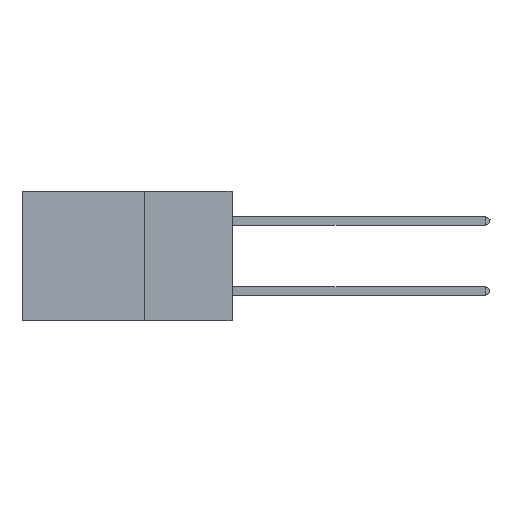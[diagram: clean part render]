
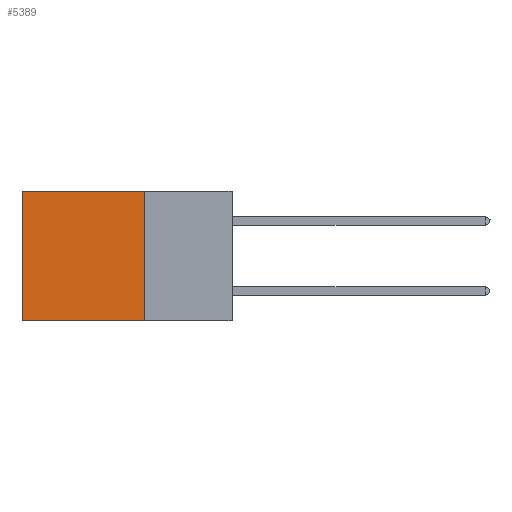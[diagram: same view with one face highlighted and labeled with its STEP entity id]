
A CAD part, left-side view. The second image highlights one B-rep face of the part: STEP entity #5389.
In plain terms, the highlighted planar face has unit normal (-1, 0, 0).
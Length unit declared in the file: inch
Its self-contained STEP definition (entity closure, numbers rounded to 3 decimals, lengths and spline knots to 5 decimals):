
#2320 = LINE ( 'NONE', #43540, #10489 ) ;
#3281 = DIRECTION ( 'NONE',  ( 0., 1., 0. ) ) ;
#3427 = FACE_OUTER_BOUND ( 'NONE', #35439, .T. ) ;
#4318 = VERTEX_POINT ( 'NONE', #36390 ) ;
#5187 = EDGE_CURVE ( 'NONE', #39572, #15517, #11845, .T. ) ;
#5389 = ADVANCED_FACE ( 'NONE', ( #3427 ), #18281, .F. ) ;
#7312 = ORIENTED_EDGE ( 'NONE', *, *, #5187, .F. ) ;
#10489 = VECTOR ( 'NONE', #17189, 39.37008 ) ;
#10857 = CARTESIAN_POINT ( 'NONE',  ( 0.2875, 0.25, -0.37 ) ) ;
#11482 = DIRECTION ( 'NONE',  ( 1., 0., 0. ) ) ;
#11845 = LINE ( 'NONE', #30617, #43500 ) ;
#12340 = AXIS2_PLACEMENT_3D ( 'NONE', #45626, #11482, #38068 ) ;
#12541 = LINE ( 'NONE', #42318, #17857 ) ;
#12564 = EDGE_CURVE ( 'NONE', #4318, #14805, #47697, .T. ) ;
#14027 = ORIENTED_EDGE ( 'NONE', *, *, #16453, .F. ) ;
#14805 = VERTEX_POINT ( 'NONE', #29355 ) ;
#15517 = VERTEX_POINT ( 'NONE', #36804 ) ;
#16453 = EDGE_CURVE ( 'NONE', #4318, #39572, #2320, .T. ) ;
#17189 = DIRECTION ( 'NONE',  ( 0., 0., -1. ) ) ;
#17857 = VECTOR ( 'NONE', #37928, 39.37008 ) ;
#18281 = PLANE ( 'NONE',  #12340 ) ;
#21557 = VECTOR ( 'NONE', #3281, 39.37008 ) ;
#23055 = EDGE_CURVE ( 'NONE', #14805, #15517, #12541, .T. ) ;
#29287 = ORIENTED_EDGE ( 'NONE', *, *, #23055, .T. ) ;
#29355 = CARTESIAN_POINT ( 'NONE',  ( 0.2875, 0.6, 0. ) ) ;
#29632 = CARTESIAN_POINT ( 'NONE',  ( 0.2875, 0.25, 0. ) ) ;
#29923 = ORIENTED_EDGE ( 'NONE', *, *, #12564, .T. ) ;
#30617 = CARTESIAN_POINT ( 'NONE',  ( 0.2875, 0.25, -0.37 ) ) ;
#35439 = EDGE_LOOP ( 'NONE', ( #29287, #7312, #14027, #29923 ) ) ;
#36390 = CARTESIAN_POINT ( 'NONE',  ( 0.2875, 0.25, 0. ) ) ;
#36804 = CARTESIAN_POINT ( 'NONE',  ( 0.2875, 0.6, -0.37 ) ) ;
#37928 = DIRECTION ( 'NONE',  ( 0., 0., -1. ) ) ;
#38068 = DIRECTION ( 'NONE',  ( 0., 0., -1. ) ) ;
#38188 = DIRECTION ( 'NONE',  ( 0., 1., 0. ) ) ;
#39572 = VERTEX_POINT ( 'NONE', #10857 ) ;
#42318 = CARTESIAN_POINT ( 'NONE',  ( 0.2875, 0.6, 0. ) ) ;
#43500 = VECTOR ( 'NONE', #38188, 39.37008 ) ;
#43540 = CARTESIAN_POINT ( 'NONE',  ( 0.2875, 0.25, 0. ) ) ;
#45626 = CARTESIAN_POINT ( 'NONE',  ( 0.2875, 0.25, 0. ) ) ;
#47697 = LINE ( 'NONE', #29632, #21557 ) ;
